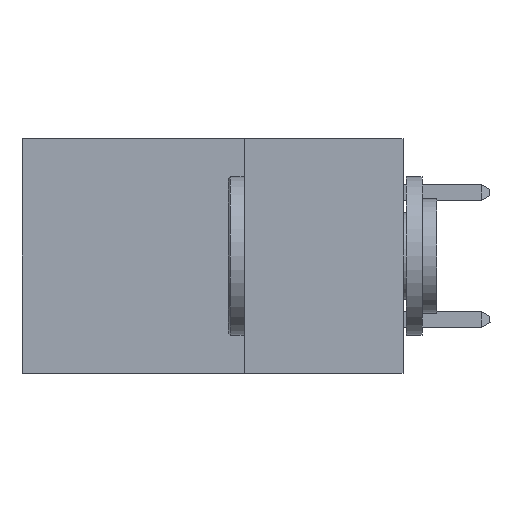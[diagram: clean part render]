
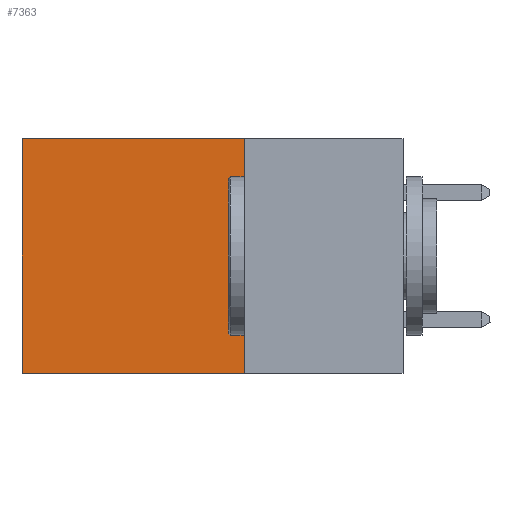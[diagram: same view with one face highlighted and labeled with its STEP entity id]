
A CAD part, left-side view. The second image highlights one B-rep face of the part: STEP entity #7363.
In plain terms, the highlighted planar face has unit normal (-1, 0, 0).
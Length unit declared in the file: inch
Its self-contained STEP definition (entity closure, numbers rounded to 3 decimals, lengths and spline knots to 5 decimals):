
#1005 = ORIENTED_EDGE ( 'NONE', *, *, #32463, .F. ) ;
#1184 = EDGE_CURVE ( 'NONE', #29713, #15284, #28588, .T. ) ;
#1604 = VECTOR ( 'NONE', #28202, 39.37008 ) ;
#1612 = PLANE ( 'NONE',  #7164 ) ;
#1729 = DIRECTION ( 'NONE',  ( 1., 0., 0. ) ) ;
#3523 = CARTESIAN_POINT ( 'NONE',  ( 0.2875, 0.6, -0.37 ) ) ;
#3889 = DIRECTION ( 'NONE',  ( 0., 0., -1. ) ) ;
#3975 = VECTOR ( 'NONE', #32827, 39.37008 ) ;
#4631 = CARTESIAN_POINT ( 'NONE',  ( 0.2875, 0.25, 0. ) ) ;
#5144 = EDGE_LOOP ( 'NONE', ( #21980, #28408, #1005, #9570 ) ) ;
#7106 = VECTOR ( 'NONE', #23608, 39.37008 ) ;
#7164 = AXIS2_PLACEMENT_3D ( 'NONE', #27136, #1729, #3889 ) ;
#7263 = VERTEX_POINT ( 'NONE', #9259 ) ;
#7363 = ADVANCED_FACE ( 'NONE', ( #10843 ), #1612, .F. ) ;
#8401 = VERTEX_POINT ( 'NONE', #23609 ) ;
#8525 = LINE ( 'NONE', #10378, #1604 ) ;
#9259 = CARTESIAN_POINT ( 'NONE',  ( 0.2875, 0.25, 0. ) ) ;
#9570 = ORIENTED_EDGE ( 'NONE', *, *, #22452, .T. ) ;
#10378 = CARTESIAN_POINT ( 'NONE',  ( 0.2875, 0.25, 0. ) ) ;
#10843 = FACE_OUTER_BOUND ( 'NONE', #5144, .T. ) ;
#15284 = VERTEX_POINT ( 'NONE', #3523 ) ;
#16699 = VECTOR ( 'NONE', #30729, 39.37008 ) ;
#17198 = CARTESIAN_POINT ( 'NONE',  ( 0.2875, 0.6, 0. ) ) ;
#21980 = ORIENTED_EDGE ( 'NONE', *, *, #1184, .T. ) ;
#22452 = EDGE_CURVE ( 'NONE', #7263, #29713, #30550, .T. ) ;
#22588 = CARTESIAN_POINT ( 'NONE',  ( 0.2875, 0.25, -0.37 ) ) ;
#23608 = DIRECTION ( 'NONE',  ( 0., 0., -1. ) ) ;
#23609 = CARTESIAN_POINT ( 'NONE',  ( 0.2875, 0.25, -0.37 ) ) ;
#24240 = LINE ( 'NONE', #22588, #3975 ) ;
#27136 = CARTESIAN_POINT ( 'NONE',  ( 0.2875, 0.25, 0. ) ) ;
#28202 = DIRECTION ( 'NONE',  ( 0., 0., -1. ) ) ;
#28408 = ORIENTED_EDGE ( 'NONE', *, *, #30339, .F. ) ;
#28588 = LINE ( 'NONE', #31340, #7106 ) ;
#29713 = VERTEX_POINT ( 'NONE', #17198 ) ;
#30339 = EDGE_CURVE ( 'NONE', #8401, #15284, #24240, .T. ) ;
#30550 = LINE ( 'NONE', #4631, #16699 ) ;
#30729 = DIRECTION ( 'NONE',  ( 0., 1., 0. ) ) ;
#31340 = CARTESIAN_POINT ( 'NONE',  ( 0.2875, 0.6, 0. ) ) ;
#32463 = EDGE_CURVE ( 'NONE', #7263, #8401, #8525, .T. ) ;
#32827 = DIRECTION ( 'NONE',  ( 0., 1., 0. ) ) ;
